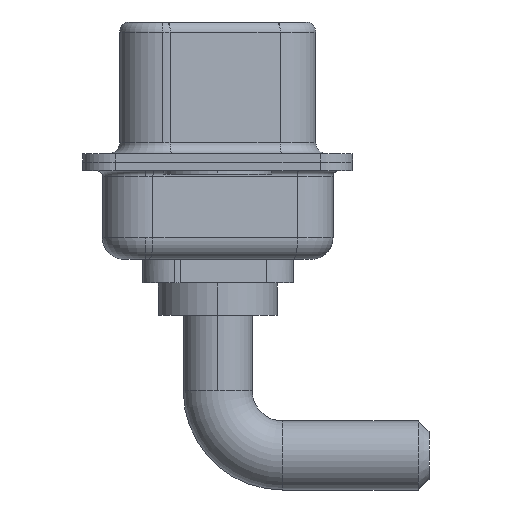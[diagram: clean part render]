
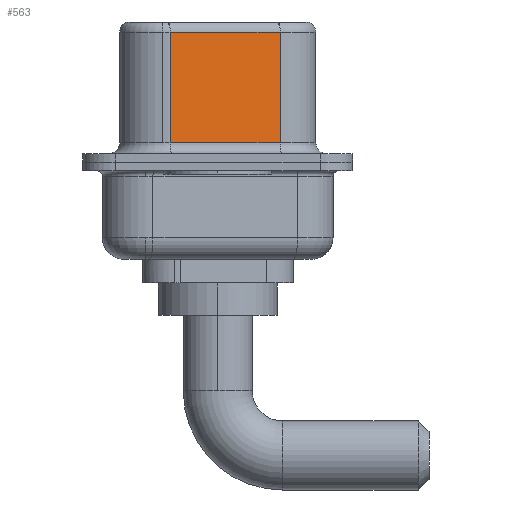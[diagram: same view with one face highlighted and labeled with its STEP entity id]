
A CAD part, left-side view. The second image highlights one B-rep face of the part: STEP entity #563.
In plain terms, the highlighted planar face has unit normal (-0.985, -0.174, 0).
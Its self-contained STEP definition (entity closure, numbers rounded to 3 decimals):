
#563 = ADVANCED_FACE ( 'NONE', ( #6517 ), #11953, .F. ) ;
#888 = LINE ( 'NONE', #14182, #13722 ) ;
#2423 = VERTEX_POINT ( 'NONE', #4690 ) ;
#3058 = CARTESIAN_POINT ( 'NONE',  ( 4.58, -2.897, 6.52 ) ) ;
#3168 = EDGE_CURVE ( 'NONE', #10173, #10929, #10952, .T. ) ;
#3485 = EDGE_CURVE ( 'NONE', #2423, #10173, #7806, .T. ) ;
#4013 = CARTESIAN_POINT ( 'NONE',  ( 3.68, 2.203, 0.9 ) ) ;
#4093 = AXIS2_PLACEMENT_3D ( 'NONE', #3058, #9708, #5504 ) ;
#4273 = DIRECTION ( 'NONE',  ( 0., 0., -1. ) ) ;
#4690 = CARTESIAN_POINT ( 'NONE',  ( 4.58, -2.897, 6.02 ) ) ;
#5448 = DIRECTION ( 'NONE',  ( 0., 0., -1. ) ) ;
#5475 = ORIENTED_EDGE ( 'NONE', *, *, #3168, .T. ) ;
#5504 = DIRECTION ( 'NONE',  ( -0.174, 0.985, 0. ) ) ;
#5559 = VECTOR ( 'NONE', #8794, 1000. ) ;
#5617 = CARTESIAN_POINT ( 'NONE',  ( 3.68, 2.203, 6.02 ) ) ;
#5666 = EDGE_CURVE ( 'NONE', #10929, #11268, #11041, .T. ) ;
#6190 = VECTOR ( 'NONE', #5448, 1000. ) ;
#6517 = FACE_OUTER_BOUND ( 'NONE', #12691, .T. ) ;
#6804 = CARTESIAN_POINT ( 'NONE',  ( 4.58, -2.897, 6.02 ) ) ;
#7033 = CARTESIAN_POINT ( 'NONE',  ( 4.58, -2.897, 0.9 ) ) ;
#7806 = LINE ( 'NONE', #6804, #11048 ) ;
#8190 = ORIENTED_EDGE ( 'NONE', *, *, #3485, .T. ) ;
#8650 = CARTESIAN_POINT ( 'NONE',  ( 4.58, -2.897, 0.9 ) ) ;
#8794 = DIRECTION ( 'NONE',  ( 0.174, -0.985, 0. ) ) ;
#9679 = EDGE_CURVE ( 'NONE', #2423, #11268, #888, .T. ) ;
#9708 = DIRECTION ( 'NONE',  ( 0.985, 0.174, 0. ) ) ;
#9798 = ORIENTED_EDGE ( 'NONE', *, *, #5666, .T. ) ;
#10014 = CARTESIAN_POINT ( 'NONE',  ( 3.68, 2.203, 6.52 ) ) ;
#10173 = VERTEX_POINT ( 'NONE', #5617 ) ;
#10929 = VERTEX_POINT ( 'NONE', #4013 ) ;
#10952 = LINE ( 'NONE', #10014, #6190 ) ;
#11041 = LINE ( 'NONE', #8650, #5559 ) ;
#11048 = VECTOR ( 'NONE', #14188, 1000. ) ;
#11268 = VERTEX_POINT ( 'NONE', #7033 ) ;
#11782 = ORIENTED_EDGE ( 'NONE', *, *, #9679, .F. ) ;
#11953 = PLANE ( 'NONE',  #4093 ) ;
#12691 = EDGE_LOOP ( 'NONE', ( #11782, #8190, #5475, #9798 ) ) ;
#13722 = VECTOR ( 'NONE', #4273, 1000. ) ;
#14182 = CARTESIAN_POINT ( 'NONE',  ( 4.58, -2.897, 6.52 ) ) ;
#14188 = DIRECTION ( 'NONE',  ( -0.174, 0.985, 0. ) ) ;
